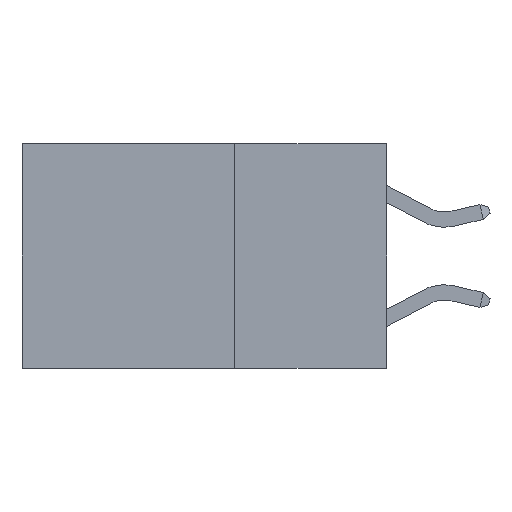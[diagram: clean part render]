
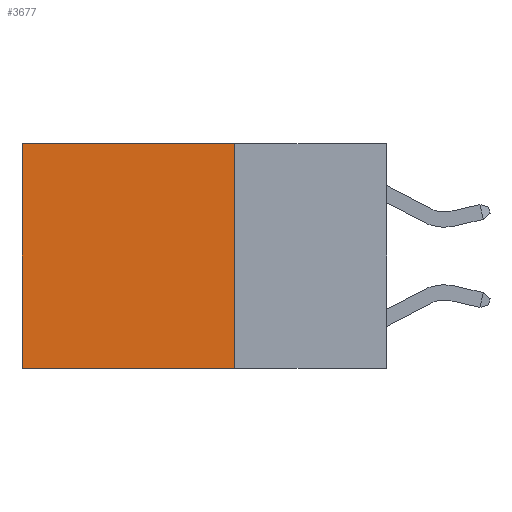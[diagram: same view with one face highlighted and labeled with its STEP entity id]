
A CAD part, left-side view. The second image highlights one B-rep face of the part: STEP entity #3677.
In plain terms, the highlighted planar face has unit normal (-1, 0, 0).
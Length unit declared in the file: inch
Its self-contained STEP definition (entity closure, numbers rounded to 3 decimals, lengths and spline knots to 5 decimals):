
#75 = DIRECTION ( 'NONE',  ( 0., 1., 0. ) ) ;
#80 = AXIS2_PLACEMENT_3D ( 'NONE', #6795, #11112, #10130 ) ;
#127 = CARTESIAN_POINT ( 'NONE',  ( 0.2625, 0.25, -0.37 ) ) ;
#230 = EDGE_CURVE ( 'NONE', #3299, #9540, #1527, .T. ) ;
#862 = VECTOR ( 'NONE', #75, 39.37008 ) ;
#883 = ORIENTED_EDGE ( 'NONE', *, *, #3471, .T. ) ;
#1023 = LINE ( 'NONE', #9749, #9912 ) ;
#1472 = CARTESIAN_POINT ( 'NONE',  ( 0.2625, 0.25, 0. ) ) ;
#1527 = LINE ( 'NONE', #3518, #5627 ) ;
#2140 = ORIENTED_EDGE ( 'NONE', *, *, #230, .F. ) ;
#2628 = DIRECTION ( 'NONE',  ( 0., 0., -1. ) ) ;
#3200 = FACE_OUTER_BOUND ( 'NONE', #8018, .T. ) ;
#3299 = VERTEX_POINT ( 'NONE', #1472 ) ;
#3471 = EDGE_CURVE ( 'NONE', #3299, #9318, #10997, .T. ) ;
#3518 = CARTESIAN_POINT ( 'NONE',  ( 0.2625, 0.25, 0. ) ) ;
#3540 = EDGE_CURVE ( 'NONE', #9540, #7597, #5524, .T. ) ;
#3677 = ADVANCED_FACE ( 'NONE', ( #3200 ), #6741, .F. ) ;
#4075 = CARTESIAN_POINT ( 'NONE',  ( 0.2625, 0.25, -0.37 ) ) ;
#4373 = CARTESIAN_POINT ( 'NONE',  ( 0.2625, 0.6, 0. ) ) ;
#4392 = EDGE_CURVE ( 'NONE', #9318, #7597, #1023, .T. ) ;
#4502 = DIRECTION ( 'NONE',  ( 0., 0., -1. ) ) ;
#4697 = CARTESIAN_POINT ( 'NONE',  ( 0.2625, 0.25, 0. ) ) ;
#5472 = VECTOR ( 'NONE', #8426, 39.37008 ) ;
#5524 = LINE ( 'NONE', #127, #862 ) ;
#5627 = VECTOR ( 'NONE', #2628, 39.37008 ) ;
#6741 = PLANE ( 'NONE',  #80 ) ;
#6795 = CARTESIAN_POINT ( 'NONE',  ( 0.2625, 0.25, 0. ) ) ;
#7597 = VERTEX_POINT ( 'NONE', #8732 ) ;
#8018 = EDGE_LOOP ( 'NONE', ( #9650, #8404, #2140, #883 ) ) ;
#8404 = ORIENTED_EDGE ( 'NONE', *, *, #3540, .F. ) ;
#8426 = DIRECTION ( 'NONE',  ( 0., 1., 0. ) ) ;
#8732 = CARTESIAN_POINT ( 'NONE',  ( 0.2625, 0.6, -0.37 ) ) ;
#9318 = VERTEX_POINT ( 'NONE', #4373 ) ;
#9540 = VERTEX_POINT ( 'NONE', #4075 ) ;
#9650 = ORIENTED_EDGE ( 'NONE', *, *, #4392, .T. ) ;
#9749 = CARTESIAN_POINT ( 'NONE',  ( 0.2625, 0.6, 0. ) ) ;
#9912 = VECTOR ( 'NONE', #4502, 39.37008 ) ;
#10130 = DIRECTION ( 'NONE',  ( 0., 0., -1. ) ) ;
#10997 = LINE ( 'NONE', #4697, #5472 ) ;
#11112 = DIRECTION ( 'NONE',  ( 1., 0., 0. ) ) ;
